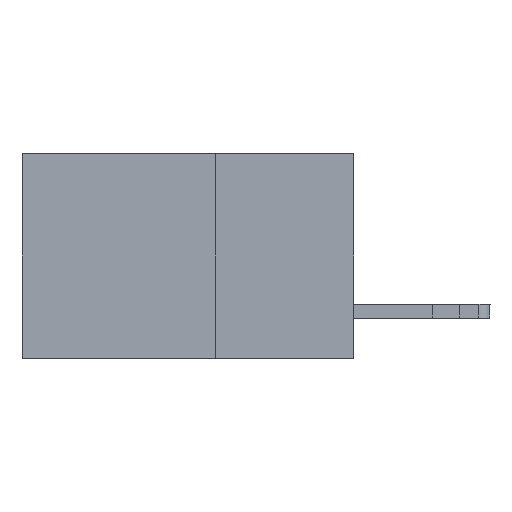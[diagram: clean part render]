
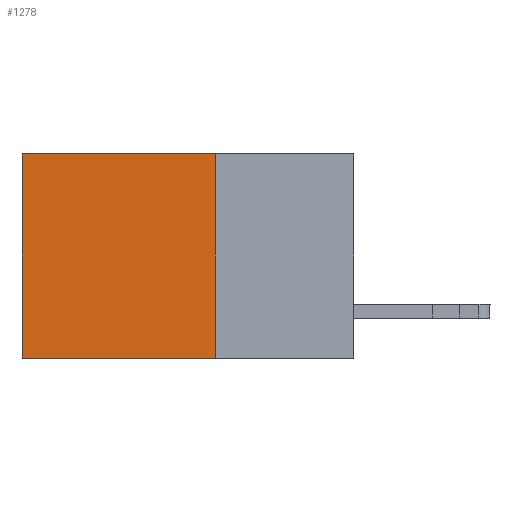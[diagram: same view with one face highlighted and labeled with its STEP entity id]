
A CAD part, left-side view. The second image highlights one B-rep face of the part: STEP entity #1278.
In plain terms, the highlighted planar face has unit normal (-1, 0, 0).
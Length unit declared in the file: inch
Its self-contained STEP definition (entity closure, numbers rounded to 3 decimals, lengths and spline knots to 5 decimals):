
#90 = EDGE_CURVE ( 'NONE', #9603, #13864, #4104, .T. ) ;
#788 = ORIENTED_EDGE ( 'NONE', *, *, #2230, .T. ) ;
#1112 = DIRECTION ( 'NONE',  ( 1., 0., 0. ) ) ;
#1278 = ADVANCED_FACE ( 'NONE', ( #7483 ), #14358, .F. ) ;
#1754 = CARTESIAN_POINT ( 'NONE',  ( 0.2875, 0.6, 0. ) ) ;
#1759 = VECTOR ( 'NONE', #12380, 39.37008 ) ;
#1954 = VECTOR ( 'NONE', #16513, 39.37008 ) ;
#2230 = EDGE_CURVE ( 'NONE', #5717, #20736, #18687, .T. ) ;
#3557 = EDGE_CURVE ( 'NONE', #13864, #20736, #19657, .T. ) ;
#4104 = LINE ( 'NONE', #7577, #1759 ) ;
#4660 = CARTESIAN_POINT ( 'NONE',  ( 0.2875, 0.25, -0.37 ) ) ;
#5717 = VERTEX_POINT ( 'NONE', #9920 ) ;
#6451 = EDGE_LOOP ( 'NONE', ( #788, #6515, #6633, #19720 ) ) ;
#6515 = ORIENTED_EDGE ( 'NONE', *, *, #3557, .F. ) ;
#6633 = ORIENTED_EDGE ( 'NONE', *, *, #90, .F. ) ;
#7483 = FACE_OUTER_BOUND ( 'NONE', #6451, .T. ) ;
#7577 = CARTESIAN_POINT ( 'NONE',  ( 0.2875, 0.25, 0. ) ) ;
#9603 = VERTEX_POINT ( 'NONE', #18433 ) ;
#9920 = CARTESIAN_POINT ( 'NONE',  ( 0.2875, 0.6, 0. ) ) ;
#11011 = CARTESIAN_POINT ( 'NONE',  ( 0.2875, 0.25, 0. ) ) ;
#12338 = VECTOR ( 'NONE', #14850, 39.37008 ) ;
#12380 = DIRECTION ( 'NONE',  ( 0., 0., -1. ) ) ;
#13116 = AXIS2_PLACEMENT_3D ( 'NONE', #11011, #1112, #17707 ) ;
#13864 = VERTEX_POINT ( 'NONE', #4660 ) ;
#13963 = CARTESIAN_POINT ( 'NONE',  ( 0.2875, 0.25, 0. ) ) ;
#14358 = PLANE ( 'NONE',  #13116 ) ;
#14818 = LINE ( 'NONE', #13963, #21612 ) ;
#14850 = DIRECTION ( 'NONE',  ( 0., 1., 0. ) ) ;
#16513 = DIRECTION ( 'NONE',  ( 0., 0., -1. ) ) ;
#16658 = EDGE_CURVE ( 'NONE', #9603, #5717, #14818, .T. ) ;
#17707 = DIRECTION ( 'NONE',  ( 0., 0., -1. ) ) ;
#18433 = CARTESIAN_POINT ( 'NONE',  ( 0.2875, 0.25, 0. ) ) ;
#18687 = LINE ( 'NONE', #1754, #1954 ) ;
#19447 = CARTESIAN_POINT ( 'NONE',  ( 0.2875, 0.6, -0.37 ) ) ;
#19657 = LINE ( 'NONE', #21422, #12338 ) ;
#19720 = ORIENTED_EDGE ( 'NONE', *, *, #16658, .T. ) ;
#20736 = VERTEX_POINT ( 'NONE', #19447 ) ;
#20753 = DIRECTION ( 'NONE',  ( 0., 1., 0. ) ) ;
#21422 = CARTESIAN_POINT ( 'NONE',  ( 0.2875, 0.25, -0.37 ) ) ;
#21612 = VECTOR ( 'NONE', #20753, 39.37008 ) ;
